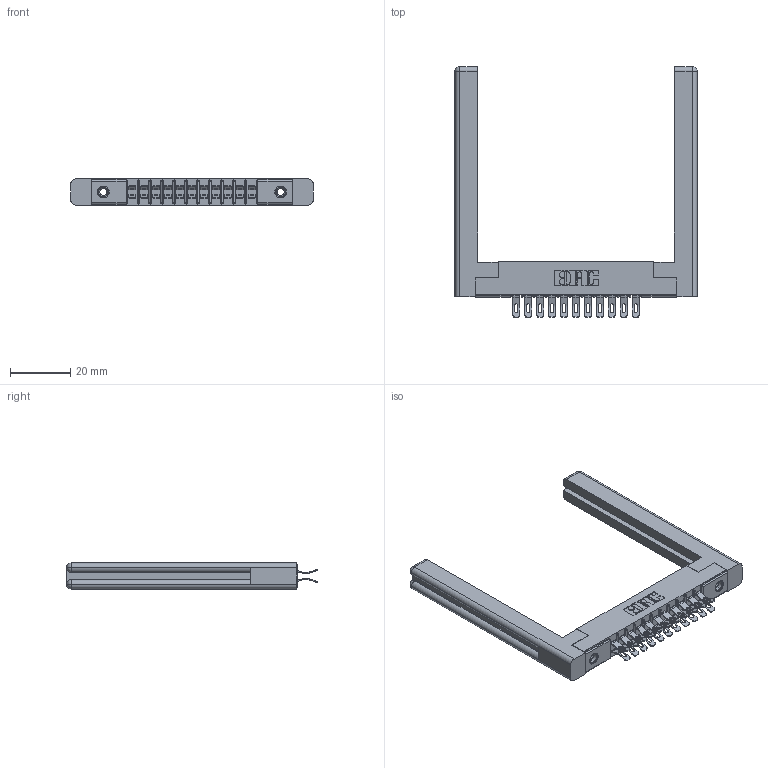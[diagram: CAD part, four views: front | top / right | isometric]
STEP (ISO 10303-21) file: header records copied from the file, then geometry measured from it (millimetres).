
FILE_DESCRIPTION (( 'STEP AP203' ), '1' );
FILE_NAME ('315-022-555-258.STEP', '2019-09-10T14:30:38', ( '' ), ( '' ), 'SwSTEP 2.0', 'SolidWorks 2016', '' );
FILE_SCHEMA (( 'CONFIG_CONTROL_DESIGN' ));
Length unit declared in the file: inch
Products named in the file (5): 305 Part_.156 Dia; 305-290-001_555; 307-220-058; 315-022-555-258; 345-250-001_345-250-001-102
Assembly tree (27 placements, depth 2):
  315-022-555-258
    305 Part_.156 Dia
    305-290-001_555  x22
    345-250-001_345-250-001-102  x2
    307-220-058  x2
Bounding box: 80.21 x 83.06 x 8.71 mm (x, y, z)
Volume: 12839.7 mm3; surface area: 14427.1 mm2
Topology: 27 solids, 27 shells, 1710 faces, 5015 edges, 3270 vertices
Faces by surface type: plane 856, cylinder 786, sphere 44, cone 12, torus 12
Entity records: 18941 total; most frequent: CARTESIAN_POINT 3168, ORIENTED_EDGE 3072, DIRECTION 3046, EDGE_CURVE 1536, VECTOR 1178, LINE 1178, VERTEX_POINT 986, AXIS2_PLACEMENT_3D 934
